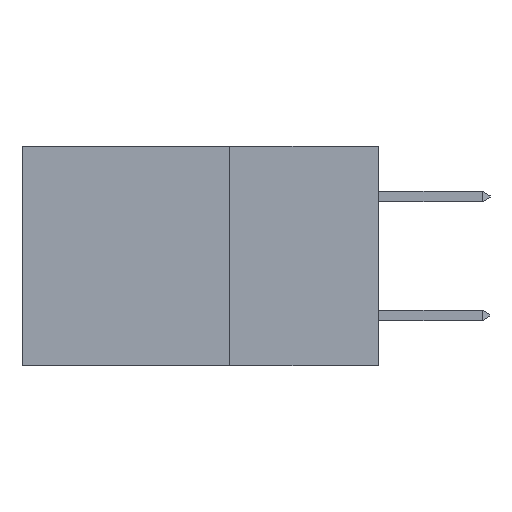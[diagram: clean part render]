
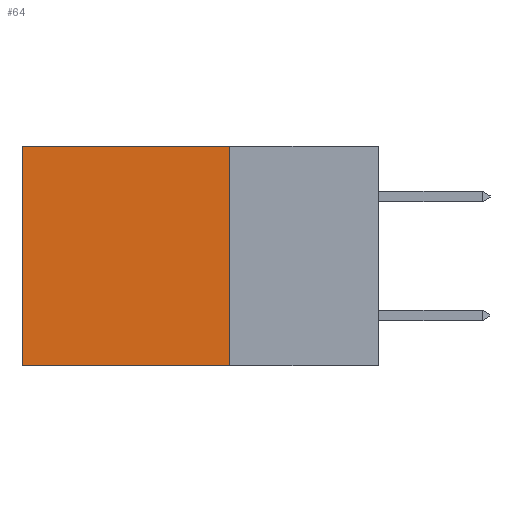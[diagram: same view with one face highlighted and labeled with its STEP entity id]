
A CAD part, left-side view. The second image highlights one B-rep face of the part: STEP entity #64.
In plain terms, the highlighted planar face has unit normal (-1, 0, 0).
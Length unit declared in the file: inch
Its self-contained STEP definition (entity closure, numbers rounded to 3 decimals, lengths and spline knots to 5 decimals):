
#55 = LINE ( 'NONE', #13706, #11905 ) ;
#64 = ADVANCED_FACE ( 'NONE', ( #6330 ), #2261, .F. ) ;
#941 = ORIENTED_EDGE ( 'NONE', *, *, #7180, .F. ) ;
#1210 = LINE ( 'NONE', #9672, #12927 ) ;
#2261 = PLANE ( 'NONE',  #8725 ) ;
#2782 = VECTOR ( 'NONE', #7047, 39.37008 ) ;
#4411 = CARTESIAN_POINT ( 'NONE',  ( 0.298, 0.6, -0.37 ) ) ;
#4912 = CARTESIAN_POINT ( 'NONE',  ( 0.298, 0.25, -0.37 ) ) ;
#5366 = DIRECTION ( 'NONE',  ( 0., 1., 0. ) ) ;
#5722 = CARTESIAN_POINT ( 'NONE',  ( 0.298, 0.25, 0. ) ) ;
#5795 = DIRECTION ( 'NONE',  ( 0., 0., -1. ) ) ;
#6330 = FACE_OUTER_BOUND ( 'NONE', #8485, .T. ) ;
#6344 = ORIENTED_EDGE ( 'NONE', *, *, #13933, .T. ) ;
#6539 = ORIENTED_EDGE ( 'NONE', *, *, #9977, .T. ) ;
#7047 = DIRECTION ( 'NONE',  ( 0., 0., -1. ) ) ;
#7180 = EDGE_CURVE ( 'NONE', #11166, #13824, #55, .T. ) ;
#8485 = EDGE_LOOP ( 'NONE', ( #6344, #941, #10854, #6539 ) ) ;
#8725 = AXIS2_PLACEMENT_3D ( 'NONE', #5722, #11614, #11117 ) ;
#9672 = CARTESIAN_POINT ( 'NONE',  ( 0.298, 0.25, 0. ) ) ;
#9977 = EDGE_CURVE ( 'NONE', #10387, #9980, #1210, .T. ) ;
#9980 = VERTEX_POINT ( 'NONE', #12921 ) ;
#10121 = LINE ( 'NONE', #14333, #12995 ) ;
#10326 = CARTESIAN_POINT ( 'NONE',  ( 0.298, 0.25, 0. ) ) ;
#10334 = EDGE_CURVE ( 'NONE', #10387, #11166, #11755, .T. ) ;
#10387 = VERTEX_POINT ( 'NONE', #10326 ) ;
#10854 = ORIENTED_EDGE ( 'NONE', *, *, #10334, .F. ) ;
#11117 = DIRECTION ( 'NONE',  ( 0., 0., -1. ) ) ;
#11166 = VERTEX_POINT ( 'NONE', #4912 ) ;
#11614 = DIRECTION ( 'NONE',  ( 1., 0., 0. ) ) ;
#11755 = LINE ( 'NONE', #12400, #2782 ) ;
#11821 = DIRECTION ( 'NONE',  ( 0., 1., 0. ) ) ;
#11905 = VECTOR ( 'NONE', #11821, 39.37008 ) ;
#12400 = CARTESIAN_POINT ( 'NONE',  ( 0.298, 0.25, 0. ) ) ;
#12921 = CARTESIAN_POINT ( 'NONE',  ( 0.298, 0.6, 0. ) ) ;
#12927 = VECTOR ( 'NONE', #5366, 39.37008 ) ;
#12995 = VECTOR ( 'NONE', #5795, 39.37008 ) ;
#13706 = CARTESIAN_POINT ( 'NONE',  ( 0.298, 0.25, -0.37 ) ) ;
#13824 = VERTEX_POINT ( 'NONE', #4411 ) ;
#13933 = EDGE_CURVE ( 'NONE', #9980, #13824, #10121, .T. ) ;
#14333 = CARTESIAN_POINT ( 'NONE',  ( 0.298, 0.6, 0. ) ) ;
